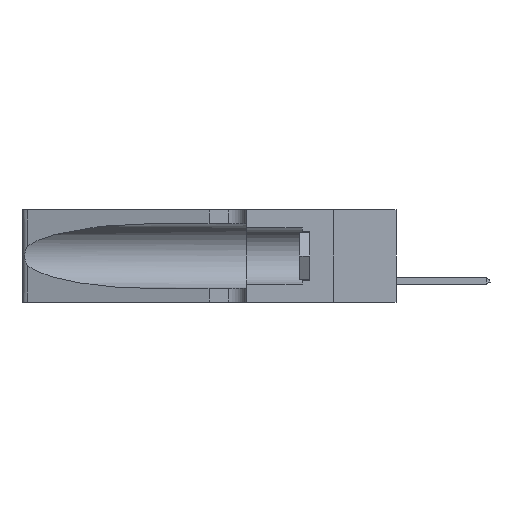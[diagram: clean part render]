
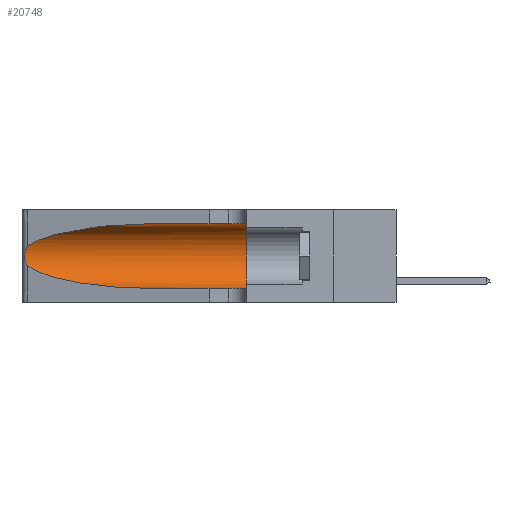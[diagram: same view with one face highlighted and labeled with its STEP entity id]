
A CAD part, left-side view. The second image highlights one B-rep face of the part: STEP entity #20748.
In plain terms, the highlighted cylindrical face has radius 3.308 mm (diameter 6.617 mm), a partial arc.
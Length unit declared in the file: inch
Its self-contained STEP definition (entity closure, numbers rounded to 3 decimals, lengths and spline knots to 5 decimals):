
#417 = CARTESIAN_POINT ( 'NONE',  ( 0.1305, 0.35, 0.05475 ) ) ;
#787 = EDGE_LOOP ( 'NONE', ( #12130, #5097, #36227, #22726, #3351, #6416 ) ) ;
#798 = CARTESIAN_POINT ( 'NONE',  ( 0.1305, 0.72297, 0.05475 ) ) ;
#1126 = CARTESIAN_POINT ( 'NONE',  ( 0.2373, 1.15595, 0.28018 ) ) ;
#1414 = CARTESIAN_POINT ( 'NONE',  ( 0.1305, 1.61858, 0.05475 ) ) ;
#1507 = CARTESIAN_POINT ( 'NONE',  ( 0.26018, 1.23835, 0.19895 ) ) ;
#2068 = CARTESIAN_POINT ( 'NONE',  ( 0.25487, 1.22718, 0.14631 ) ) ;
#2959 = CYLINDRICAL_SURFACE ( 'NONE', #17573, 0.13025 ) ;
#3351 = ORIENTED_EDGE ( 'NONE', *, *, #17783, .F. ) ;
#3997 = CARTESIAN_POINT ( 'NONE',  ( 0.25487, 1.22718, 0.14631 ) ) ;
#4215 = CARTESIAN_POINT ( 'NONE',  ( 0.1305, 0.35, 0.31525 ) ) ;
#4839 = VECTOR ( 'NONE', #6555, 39.37008 ) ;
#5097 = ORIENTED_EDGE ( 'NONE', *, *, #19500, .T. ) ;
#5842 = CARTESIAN_POINT ( 'NONE',  ( 0.1305, 1.61858, 0.185 ) ) ;
#5989 = CARTESIAN_POINT ( 'NONE',  ( 0.1305, 0.72297, 0.31525 ) ) ;
#6416 = ORIENTED_EDGE ( 'NONE', *, *, #9046, .F. ) ;
#6555 = DIRECTION ( 'NONE',  ( 0., -1., 0. ) ) ;
#6656 = DIRECTION ( 'NONE',  ( 0., 1., 0. ) ) ;
#7038 = CARTESIAN_POINT ( 'NONE',  ( 0.25854, 1.2359, 0.20912 ) ) ;
#7051 = CARTESIAN_POINT ( 'NONE',  ( 0.1305, 0.72297, 0.31525 ) ) ;
#7082 = B_SPLINE_CURVE_WITH_KNOTS ( 'NONE', 3,
 ( #10356, #24240, #7287, #12941, #7038, #1507, #7164, #21011, #26824, #9994, #29608, #32401, #21277, #24366 ),
 .UNSPECIFIED., .F., .F.,
 ( 4, 2, 2, 2, 2, 2, 4 ),
 ( 0., 0.00027, 0.00053, 0.00107, 0.0016, 0.00187, 0.00214 ),
 .UNSPECIFIED. ) ;
#7164 = CARTESIAN_POINT ( 'NONE',  ( 0.26075, 1.23896, 0.19203 ) ) ;
#7287 = CARTESIAN_POINT ( 'NONE',  ( 0.25639, 1.23184, 0.21858 ) ) ;
#9046 = EDGE_CURVE ( 'NONE', #26002, #32633, #19071, .T. ) ;
#9586 = CARTESIAN_POINT ( 'NONE',  ( 0.25487, 1.22718, 0.22369 ) ) ;
#9993 = CARTESIAN_POINT ( 'NONE',  ( 0.1305, 0.35, 0.185 ) ) ;
#9994 = CARTESIAN_POINT ( 'NONE',  ( 0.25856, 1.23593, 0.16098 ) ) ;
#10356 = CARTESIAN_POINT ( 'NONE',  ( 0.25487, 1.22718, 0.22369 ) ) ;
#10464 = VERTEX_POINT ( 'NONE', #26254 ) ;
#11622 = EDGE_CURVE ( 'NONE', #10464, #29498, #21958, .T. ) ;
#12000 = EDGE_CURVE ( 'NONE', #25017, #10464, #33113, .T. ) ;
#12130 = ORIENTED_EDGE ( 'NONE', *, *, #18908, .T. ) ;
#12941 = CARTESIAN_POINT ( 'NONE',  ( 0.25787, 1.23484, 0.2124 ) ) ;
#15656 =( BOUNDED_CURVE ( )  B_SPLINE_CURVE ( 3, ( #5989, #23970, #1126, #9586 ),
 .UNSPECIFIED., .F., .T. ) 
 B_SPLINE_CURVE_WITH_KNOTS ( ( 4, 4 ),
 ( 1.5708, 2.84003 ),
 .UNSPECIFIED. ) 
 CURVE ( )  GEOMETRIC_REPRESENTATION_ITEM ( )  RATIONAL_B_SPLINE_CURVE ( ( 1., 0.87, 0.87, 1. ) ) 
 REPRESENTATION_ITEM ( '' )  );
#16854 = VERTEX_POINT ( 'NONE', #26513 ) ;
#17030 = FACE_OUTER_BOUND ( 'NONE', #787, .T. ) ;
#17140 = DIRECTION ( 'NONE',  ( 0., 0., -1. ) ) ;
#17538 = DIRECTION ( 'NONE',  ( 0., -1., 0. ) ) ;
#17573 = AXIS2_PLACEMENT_3D ( 'NONE', #5842, #33878, #17140 ) ;
#17615 = CARTESIAN_POINT ( 'NONE',  ( 0.18966, 0.96281, 0.05475 ) ) ;
#17783 = EDGE_CURVE ( 'NONE', #32633, #29498, #35596, .T. ) ;
#18673 = VECTOR ( 'NONE', #17538, 39.37008 ) ;
#18908 = EDGE_CURVE ( 'NONE', #26002, #16854, #15656, .T. ) ;
#19071 = LINE ( 'NONE', #26291, #18673 ) ;
#19378 = DIRECTION ( 'NONE',  ( 0., 0., 1. ) ) ;
#19500 = EDGE_CURVE ( 'NONE', #16854, #25017, #7082, .T. ) ;
#20748 = ADVANCED_FACE ( 'NONE', ( #17030 ), #2959, .F. ) ;
#21011 = CARTESIAN_POINT ( 'NONE',  ( 0.26075, 1.23896, 0.178 ) ) ;
#21277 = CARTESIAN_POINT ( 'NONE',  ( 0.25555, 1.22993, 0.14849 ) ) ;
#21958 = LINE ( 'NONE', #1414, #4839 ) ;
#22726 = ORIENTED_EDGE ( 'NONE', *, *, #11622, .T. ) ;
#23970 = CARTESIAN_POINT ( 'NONE',  ( 0.18966, 0.96281, 0.31525 ) ) ;
#24240 = CARTESIAN_POINT ( 'NONE',  ( 0.25555, 1.22994, 0.2215 ) ) ;
#24366 = CARTESIAN_POINT ( 'NONE',  ( 0.25487, 1.22718, 0.14631 ) ) ;
#25017 = VERTEX_POINT ( 'NONE', #2068 ) ;
#26002 = VERTEX_POINT ( 'NONE', #7051 ) ;
#26254 = CARTESIAN_POINT ( 'NONE',  ( 0.1305, 0.72297, 0.05475 ) ) ;
#26291 = CARTESIAN_POINT ( 'NONE',  ( 0.1305, 1.61858, 0.31525 ) ) ;
#26513 = CARTESIAN_POINT ( 'NONE',  ( 0.25487, 1.22718, 0.22369 ) ) ;
#26824 = CARTESIAN_POINT ( 'NONE',  ( 0.26017, 1.23833, 0.17102 ) ) ;
#29267 = CARTESIAN_POINT ( 'NONE',  ( 0.2373, 1.15595, 0.08982 ) ) ;
#29498 = VERTEX_POINT ( 'NONE', #417 ) ;
#29608 = CARTESIAN_POINT ( 'NONE',  ( 0.25789, 1.23486, 0.15765 ) ) ;
#30684 = AXIS2_PLACEMENT_3D ( 'NONE', #9993, #6656, #19378 ) ;
#32401 = CARTESIAN_POINT ( 'NONE',  ( 0.25639, 1.23186, 0.15144 ) ) ;
#32633 = VERTEX_POINT ( 'NONE', #4215 ) ;
#33113 =( BOUNDED_CURVE ( )  B_SPLINE_CURVE ( 3, ( #3997, #29267, #17615, #798 ),
 .UNSPECIFIED., .F., .T. ) 
 B_SPLINE_CURVE_WITH_KNOTS ( ( 4, 4 ),
 ( 3.44316, 4.71239 ),
 .UNSPECIFIED. ) 
 CURVE ( )  GEOMETRIC_REPRESENTATION_ITEM ( )  RATIONAL_B_SPLINE_CURVE ( ( 1., 0.87, 0.87, 1. ) ) 
 REPRESENTATION_ITEM ( '' )  );
#33878 = DIRECTION ( 'NONE',  ( 0., -1., 0. ) ) ;
#35596 = CIRCLE ( 'NONE', #30684, 0.13025 ) ;
#36227 = ORIENTED_EDGE ( 'NONE', *, *, #12000, .T. ) ;
